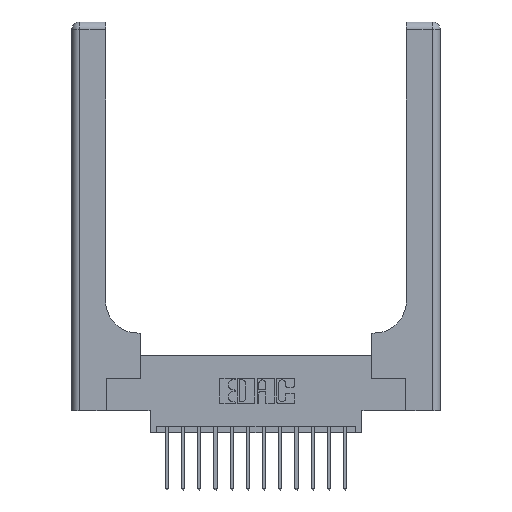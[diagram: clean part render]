
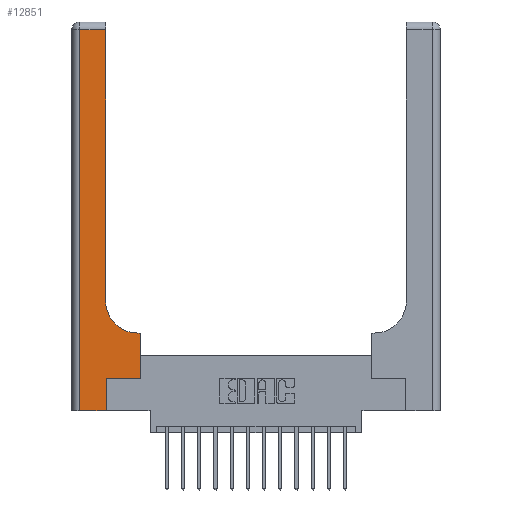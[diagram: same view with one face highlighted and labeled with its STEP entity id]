
A CAD part, top view. The second image highlights one B-rep face of the part: STEP entity #12851.
In plain terms, the highlighted planar face has unit normal (0, 0, 1).
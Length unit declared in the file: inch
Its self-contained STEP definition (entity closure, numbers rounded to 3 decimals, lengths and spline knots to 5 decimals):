
#482 = DIRECTION ( 'NONE',  ( 0., 0., -1. ) ) ;
#951 = EDGE_CURVE ( 'NONE', #7195, #10569, #3344, .T. ) ;
#1070 = DIRECTION ( 'NONE',  ( 1., 0., 0. ) ) ;
#1183 = AXIS2_PLACEMENT_3D ( 'NONE', #3352, #482, #16545 ) ;
#1444 = VERTEX_POINT ( 'NONE', #12849 ) ;
#1500 = CARTESIAN_POINT ( 'NONE',  ( 0.26, 0.6, 0.37 ) ) ;
#1515 = DIRECTION ( 'NONE',  ( 0., 1., 0. ) ) ;
#1747 = LINE ( 'NONE', #4620, #8183 ) ;
#1770 = VECTOR ( 'NONE', #13014, 39.37008 ) ;
#1899 = DIRECTION ( 'NONE',  ( 0., 1., 0. ) ) ;
#2245 = CARTESIAN_POINT ( 'NONE',  ( 0., 0., 0.37 ) ) ;
#2409 = LINE ( 'NONE', #2245, #5784 ) ;
#3164 = ORIENTED_EDGE ( 'NONE', *, *, #9514, .T. ) ;
#3344 = LINE ( 'NONE', #7539, #12154 ) ;
#3352 = CARTESIAN_POINT ( 'NONE',  ( 0.51, 0.85, 0.37 ) ) ;
#3355 = DIRECTION ( 'NONE',  ( 0., 0., -1. ) ) ;
#3507 = CARTESIAN_POINT ( 'NONE',  ( 0.265, 0.25, 0.37 ) ) ;
#3820 = ORIENTED_EDGE ( 'NONE', *, *, #5703, .T. ) ;
#4044 = LINE ( 'NONE', #4387, #8682 ) ;
#4387 = CARTESIAN_POINT ( 'NONE',  ( 0.528, 0.25, 0.37 ) ) ;
#4415 = DIRECTION ( 'NONE',  ( -1., 0., 0. ) ) ;
#4435 = DIRECTION ( 'NONE',  ( 0., 1., 0. ) ) ;
#4476 = EDGE_CURVE ( 'NONE', #6271, #7131, #1747, .T. ) ;
#4620 = CARTESIAN_POINT ( 'NONE',  ( 0.265, 0., 0.37 ) ) ;
#4668 = ORIENTED_EDGE ( 'NONE', *, *, #951, .T. ) ;
#4830 = LINE ( 'NONE', #12846, #1770 ) ;
#5321 = ORIENTED_EDGE ( 'NONE', *, *, #8731, .T. ) ;
#5538 = LINE ( 'NONE', #16405, #12654 ) ;
#5703 = EDGE_CURVE ( 'NONE', #8919, #9092, #9509, .T. ) ;
#5724 = LINE ( 'NONE', #1500, #15345 ) ;
#5750 = VERTEX_POINT ( 'NONE', #6986 ) ;
#5784 = VECTOR ( 'NONE', #1070, 39.37008 ) ;
#5942 = ORIENTED_EDGE ( 'NONE', *, *, #11655, .T. ) ;
#5959 = ORIENTED_EDGE ( 'NONE', *, *, #8303, .T. ) ;
#6022 = ORIENTED_EDGE ( 'NONE', *, *, #15154, .T. ) ;
#6262 = EDGE_CURVE ( 'NONE', #12329, #1444, #5724, .T. ) ;
#6271 = VERTEX_POINT ( 'NONE', #7922 ) ;
#6290 = CARTESIAN_POINT ( 'NONE',  ( 0.26, 2.94, 0.37 ) ) ;
#6845 = ORIENTED_EDGE ( 'NONE', *, *, #4476, .T. ) ;
#6930 = EDGE_LOOP ( 'NONE', ( #4668, #3164, #3820, #5959, #6845, #5321, #6022, #9820, #5942 ) ) ;
#6962 = DIRECTION ( 'NONE',  ( -1., 0., 0. ) ) ;
#6986 = CARTESIAN_POINT ( 'NONE',  ( 0.528, 0.25, 0.37 ) ) ;
#7131 = VERTEX_POINT ( 'NONE', #3507 ) ;
#7195 = VERTEX_POINT ( 'NONE', #8139 ) ;
#7539 = CARTESIAN_POINT ( 'NONE',  ( 0.26, 3., 0.37 ) ) ;
#7922 = CARTESIAN_POINT ( 'NONE',  ( 0.265, 0., 0.37 ) ) ;
#7950 = VECTOR ( 'NONE', #10031, 39.37008 ) ;
#8139 = CARTESIAN_POINT ( 'NONE',  ( 0.26, 0.85, 0.37 ) ) ;
#8183 = VECTOR ( 'NONE', #4435, 39.37008 ) ;
#8214 = CARTESIAN_POINT ( 'NONE',  ( 0.06, 2.94, 0.37 ) ) ;
#8303 = EDGE_CURVE ( 'NONE', #9092, #6271, #2409, .T. ) ;
#8455 = PLANE ( 'NONE',  #15929 ) ;
#8682 = VECTOR ( 'NONE', #1515, 39.37008 ) ;
#8731 = EDGE_CURVE ( 'NONE', #7131, #5750, #4830, .T. ) ;
#8919 = VERTEX_POINT ( 'NONE', #8214 ) ;
#9092 = VERTEX_POINT ( 'NONE', #17100 ) ;
#9398 = CARTESIAN_POINT ( 'NONE',  ( 0.528, 0.6, 0.37 ) ) ;
#9509 = LINE ( 'NONE', #13939, #7950 ) ;
#9514 = EDGE_CURVE ( 'NONE', #10569, #8919, #5538, .T. ) ;
#9820 = ORIENTED_EDGE ( 'NONE', *, *, #6262, .T. ) ;
#10031 = DIRECTION ( 'NONE',  ( 0., -1., 0. ) ) ;
#10137 = FACE_OUTER_BOUND ( 'NONE', #6930, .T. ) ;
#10569 = VERTEX_POINT ( 'NONE', #6290 ) ;
#11655 = EDGE_CURVE ( 'NONE', #1444, #7195, #14570, .T. ) ;
#12154 = VECTOR ( 'NONE', #1899, 39.37008 ) ;
#12329 = VERTEX_POINT ( 'NONE', #9398 ) ;
#12471 = DIRECTION ( 'NONE',  ( -1., 0., 0. ) ) ;
#12654 = VECTOR ( 'NONE', #12471, 39.37008 ) ;
#12846 = CARTESIAN_POINT ( 'NONE',  ( 0.265, 0.25, 0.37 ) ) ;
#12849 = CARTESIAN_POINT ( 'NONE',  ( 0.51, 0.6, 0.37 ) ) ;
#12851 = ADVANCED_FACE ( 'NONE', ( #10137 ), #8455, .F. ) ;
#13014 = DIRECTION ( 'NONE',  ( 1., 0., 0. ) ) ;
#13939 = CARTESIAN_POINT ( 'NONE',  ( 0.06, 3., 0.37 ) ) ;
#14570 = CIRCLE ( 'NONE', #1183, 0.25 ) ;
#15154 = EDGE_CURVE ( 'NONE', #5750, #12329, #4044, .T. ) ;
#15345 = VECTOR ( 'NONE', #6962, 39.37008 ) ;
#15929 = AXIS2_PLACEMENT_3D ( 'NONE', #16902, #3355, #4415 ) ;
#16405 = CARTESIAN_POINT ( 'NONE',  ( 0., 2.94, 0.37 ) ) ;
#16545 = DIRECTION ( 'NONE',  ( 1., 0., 0. ) ) ;
#16902 = CARTESIAN_POINT ( 'NONE',  ( 0., 3., 0.37 ) ) ;
#17100 = CARTESIAN_POINT ( 'NONE',  ( 0.06, 0., 0.37 ) ) ;
